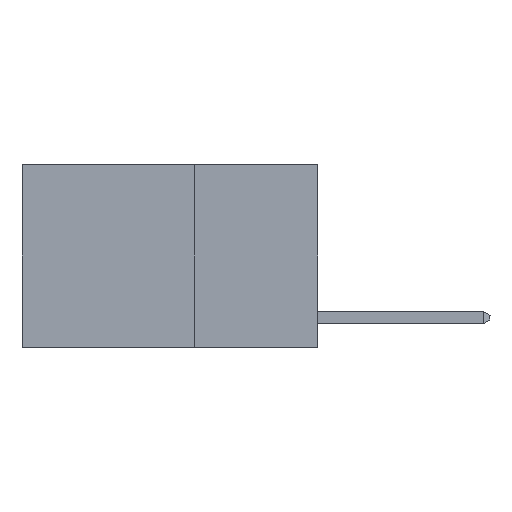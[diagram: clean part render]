
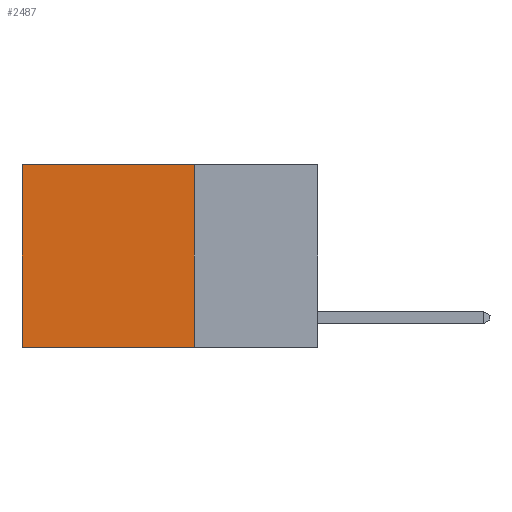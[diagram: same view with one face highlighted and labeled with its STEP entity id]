
A CAD part, left-side view. The second image highlights one B-rep face of the part: STEP entity #2487.
In plain terms, the highlighted planar face has unit normal (-1, 0, 0).
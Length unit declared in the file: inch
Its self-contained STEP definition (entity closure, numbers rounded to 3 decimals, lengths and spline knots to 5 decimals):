
#2066 = CARTESIAN_POINT ( 'NONE',  ( 0.2625, 0.6, 0. ) ) ;
#2364 = DIRECTION ( 'NONE',  ( 0., 1., 0. ) ) ;
#2447 = VERTEX_POINT ( 'NONE', #14282 ) ;
#2487 = ADVANCED_FACE ( 'NONE', ( #11595 ), #20831, .F. ) ;
#3466 = EDGE_CURVE ( 'NONE', #10345, #13052, #20905, .T. ) ;
#5070 = CARTESIAN_POINT ( 'NONE',  ( 0.2625, 0.25, 0. ) ) ;
#5102 = VECTOR ( 'NONE', #2364, 39.37008 ) ;
#6393 = CARTESIAN_POINT ( 'NONE',  ( 0.2625, 0.25, 0. ) ) ;
#6994 = LINE ( 'NONE', #2066, #17701 ) ;
#7126 = LINE ( 'NONE', #8575, #5102 ) ;
#8048 = DIRECTION ( 'NONE',  ( 1., 0., 0. ) ) ;
#8448 = DIRECTION ( 'NONE',  ( 0., 1., 0. ) ) ;
#8575 = CARTESIAN_POINT ( 'NONE',  ( 0.2625, 0.25, -0.37 ) ) ;
#9024 = CARTESIAN_POINT ( 'NONE',  ( 0.2625, 0.25, 0. ) ) ;
#9406 = DIRECTION ( 'NONE',  ( 0., 0., -1. ) ) ;
#9425 = AXIS2_PLACEMENT_3D ( 'NONE', #18606, #8048, #22989 ) ;
#9566 = VECTOR ( 'NONE', #9406, 39.37008 ) ;
#9665 = ORIENTED_EDGE ( 'NONE', *, *, #21631, .T. ) ;
#10345 = VERTEX_POINT ( 'NONE', #9024 ) ;
#11595 = FACE_OUTER_BOUND ( 'NONE', #20284, .T. ) ;
#11844 = ORIENTED_EDGE ( 'NONE', *, *, #3466, .F. ) ;
#11952 = CARTESIAN_POINT ( 'NONE',  ( 0.2625, 0.6, -0.37 ) ) ;
#12465 = EDGE_CURVE ( 'NONE', #13052, #26183, #7126, .T. ) ;
#13052 = VERTEX_POINT ( 'NONE', #21601 ) ;
#14282 = CARTESIAN_POINT ( 'NONE',  ( 0.2625, 0.6, 0. ) ) ;
#17701 = VECTOR ( 'NONE', #19197, 39.37008 ) ;
#18102 = ORIENTED_EDGE ( 'NONE', *, *, #12465, .F. ) ;
#18376 = VECTOR ( 'NONE', #8448, 39.37008 ) ;
#18606 = CARTESIAN_POINT ( 'NONE',  ( 0.2625, 0.25, 0. ) ) ;
#19197 = DIRECTION ( 'NONE',  ( 0., 0., -1. ) ) ;
#20284 = EDGE_LOOP ( 'NONE', ( #25106, #18102, #11844, #9665 ) ) ;
#20831 = PLANE ( 'NONE',  #9425 ) ;
#20905 = LINE ( 'NONE', #5070, #9566 ) ;
#21601 = CARTESIAN_POINT ( 'NONE',  ( 0.2625, 0.25, -0.37 ) ) ;
#21630 = EDGE_CURVE ( 'NONE', #2447, #26183, #6994, .T. ) ;
#21631 = EDGE_CURVE ( 'NONE', #10345, #2447, #23399, .T. ) ;
#22989 = DIRECTION ( 'NONE',  ( 0., 0., -1. ) ) ;
#23399 = LINE ( 'NONE', #6393, #18376 ) ;
#25106 = ORIENTED_EDGE ( 'NONE', *, *, #21630, .T. ) ;
#26183 = VERTEX_POINT ( 'NONE', #11952 ) ;
